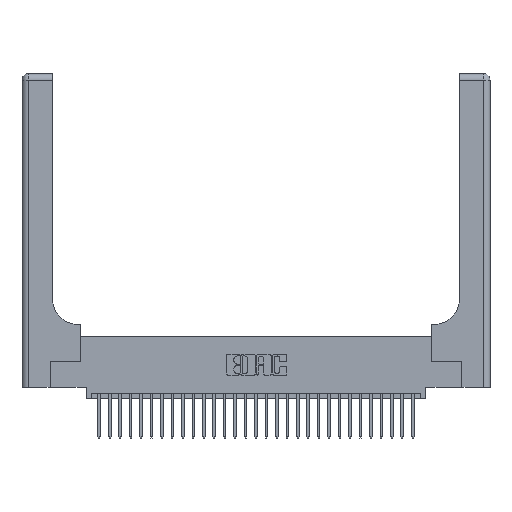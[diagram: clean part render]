
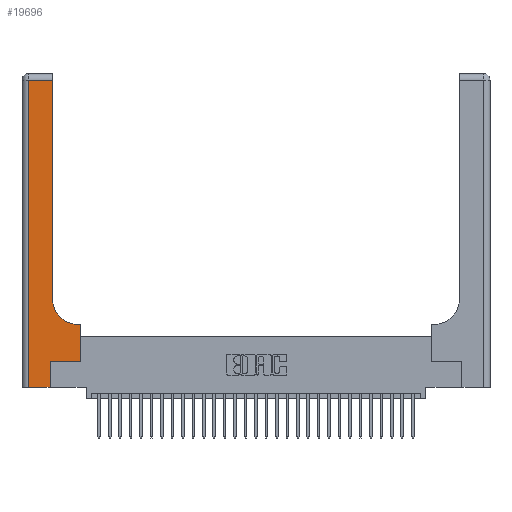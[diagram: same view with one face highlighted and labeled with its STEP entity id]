
A CAD part, top view. The second image highlights one B-rep face of the part: STEP entity #19696.
In plain terms, the highlighted planar face has unit normal (0, 0, 1).
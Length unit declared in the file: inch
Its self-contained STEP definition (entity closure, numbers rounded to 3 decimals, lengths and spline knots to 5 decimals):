
#331 = CARTESIAN_POINT ( 'NONE',  ( 0.269, 0., 0.37 ) ) ;
#370 = FACE_OUTER_BOUND ( 'NONE', #11109, .T. ) ;
#678 = CARTESIAN_POINT ( 'NONE',  ( 0.5415, 0.6, 0.37 ) ) ;
#966 = DIRECTION ( 'NONE',  ( -1., 0., 0. ) ) ;
#1304 = VECTOR ( 'NONE', #3362, 39.37008 ) ;
#1441 = CARTESIAN_POINT ( 'NONE',  ( 0.06, 0., 0.37 ) ) ;
#1994 = DIRECTION ( 'NONE',  ( 0., -1., 0. ) ) ;
#2653 = CIRCLE ( 'NONE', #16858, 0.25 ) ;
#2916 = CARTESIAN_POINT ( 'NONE',  ( 0.269, 0.25, 0.37 ) ) ;
#3362 = DIRECTION ( 'NONE',  ( 0., 1., 0. ) ) ;
#3398 = CARTESIAN_POINT ( 'NONE',  ( 0.2915, 0.6, 0.37 ) ) ;
#4058 = CARTESIAN_POINT ( 'NONE',  ( 0., 0., 0.37 ) ) ;
#4852 = DIRECTION ( 'NONE',  ( 0., 0., -1. ) ) ;
#5657 = LINE ( 'NONE', #11842, #16652 ) ;
#6218 = PLANE ( 'NONE',  #8424 ) ;
#6545 = CARTESIAN_POINT ( 'NONE',  ( 0.5585, 0.25, 0.37 ) ) ;
#7161 = EDGE_CURVE ( 'NONE', #25264, #28303, #5657, .T. ) ;
#7382 = ORIENTED_EDGE ( 'NONE', *, *, #10110, .T. ) ;
#7526 = DIRECTION ( 'NONE',  ( 1., 0., 0. ) ) ;
#7592 = ORIENTED_EDGE ( 'NONE', *, *, #19439, .T. ) ;
#7774 = VERTEX_POINT ( 'NONE', #17921 ) ;
#8424 = AXIS2_PLACEMENT_3D ( 'NONE', #8442, #25312, #966 ) ;
#8442 = CARTESIAN_POINT ( 'NONE',  ( 0., 3., 0.37 ) ) ;
#8927 = ORIENTED_EDGE ( 'NONE', *, *, #16326, .T. ) ;
#9055 = VERTEX_POINT ( 'NONE', #1441 ) ;
#9857 = LINE ( 'NONE', #15215, #21924 ) ;
#10110 = EDGE_CURVE ( 'NONE', #13024, #7774, #29680, .T. ) ;
#11109 = EDGE_LOOP ( 'NONE', ( #23827, #28354, #7592, #17766, #14988, #7382, #8927, #22747, #18179 ) ) ;
#11842 = CARTESIAN_POINT ( 'NONE',  ( 0., 2.94, 0.37 ) ) ;
#12074 = CARTESIAN_POINT ( 'NONE',  ( 0.2915, 2.94, 0.37 ) ) ;
#12163 = VECTOR ( 'NONE', #13843, 39.37008 ) ;
#12184 = VECTOR ( 'NONE', #13422, 39.37008 ) ;
#13024 = VERTEX_POINT ( 'NONE', #2916 ) ;
#13152 = CARTESIAN_POINT ( 'NONE',  ( 0.2915, 3., 0.37 ) ) ;
#13422 = DIRECTION ( 'NONE',  ( -1., 0., 0. ) ) ;
#13843 = DIRECTION ( 'NONE',  ( 1., 0., 0. ) ) ;
#14138 = VERTEX_POINT ( 'NONE', #678 ) ;
#14988 = ORIENTED_EDGE ( 'NONE', *, *, #18577, .T. ) ;
#15176 = EDGE_CURVE ( 'NONE', #14138, #17523, #2653, .T. ) ;
#15215 = CARTESIAN_POINT ( 'NONE',  ( 0.269, 0., 0.37 ) ) ;
#15914 = VERTEX_POINT ( 'NONE', #331 ) ;
#16326 = EDGE_CURVE ( 'NONE', #7774, #21182, #16401, .T. ) ;
#16362 = EDGE_CURVE ( 'NONE', #17523, #25264, #22003, .T. ) ;
#16401 = LINE ( 'NONE', #6545, #26165 ) ;
#16562 = VECTOR ( 'NONE', #26890, 39.37008 ) ;
#16652 = VECTOR ( 'NONE', #21120, 39.37008 ) ;
#16831 = EDGE_CURVE ( 'NONE', #21182, #14138, #18631, .T. ) ;
#16858 = AXIS2_PLACEMENT_3D ( 'NONE', #30509, #4852, #7526 ) ;
#17083 = EDGE_CURVE ( 'NONE', #9055, #15914, #29507, .T. ) ;
#17523 = VERTEX_POINT ( 'NONE', #18868 ) ;
#17766 = ORIENTED_EDGE ( 'NONE', *, *, #17083, .T. ) ;
#17921 = CARTESIAN_POINT ( 'NONE',  ( 0.5585, 0.25, 0.37 ) ) ;
#18179 = ORIENTED_EDGE ( 'NONE', *, *, #15176, .T. ) ;
#18566 = CARTESIAN_POINT ( 'NONE',  ( 0.06, 2.94, 0.37 ) ) ;
#18577 = EDGE_CURVE ( 'NONE', #15914, #13024, #9857, .T. ) ;
#18631 = LINE ( 'NONE', #3398, #12184 ) ;
#18649 = CARTESIAN_POINT ( 'NONE',  ( 0.06, 3., 0.37 ) ) ;
#18868 = CARTESIAN_POINT ( 'NONE',  ( 0.2915, 0.85, 0.37 ) ) ;
#19439 = EDGE_CURVE ( 'NONE', #28303, #9055, #28651, .T. ) ;
#19696 = ADVANCED_FACE ( 'NONE', ( #370 ), #6218, .F. ) ;
#20177 = CARTESIAN_POINT ( 'NONE',  ( 0.269, 0.25, 0.37 ) ) ;
#20387 = VECTOR ( 'NONE', #1994, 39.37008 ) ;
#21100 = DIRECTION ( 'NONE',  ( 0., 1., 0. ) ) ;
#21120 = DIRECTION ( 'NONE',  ( -1., 0., 0. ) ) ;
#21182 = VERTEX_POINT ( 'NONE', #26365 ) ;
#21924 = VECTOR ( 'NONE', #27083, 39.37008 ) ;
#22003 = LINE ( 'NONE', #13152, #1304 ) ;
#22747 = ORIENTED_EDGE ( 'NONE', *, *, #16831, .T. ) ;
#23827 = ORIENTED_EDGE ( 'NONE', *, *, #16362, .T. ) ;
#25264 = VERTEX_POINT ( 'NONE', #12074 ) ;
#25312 = DIRECTION ( 'NONE',  ( 0., 0., -1. ) ) ;
#26165 = VECTOR ( 'NONE', #21100, 39.37008 ) ;
#26365 = CARTESIAN_POINT ( 'NONE',  ( 0.5585, 0.6, 0.37 ) ) ;
#26890 = DIRECTION ( 'NONE',  ( 1., 0., 0. ) ) ;
#27083 = DIRECTION ( 'NONE',  ( 0., 1., 0. ) ) ;
#28303 = VERTEX_POINT ( 'NONE', #18566 ) ;
#28354 = ORIENTED_EDGE ( 'NONE', *, *, #7161, .T. ) ;
#28651 = LINE ( 'NONE', #18649, #20387 ) ;
#29507 = LINE ( 'NONE', #4058, #12163 ) ;
#29680 = LINE ( 'NONE', #20177, #16562 ) ;
#30509 = CARTESIAN_POINT ( 'NONE',  ( 0.5415, 0.85, 0.37 ) ) ;
